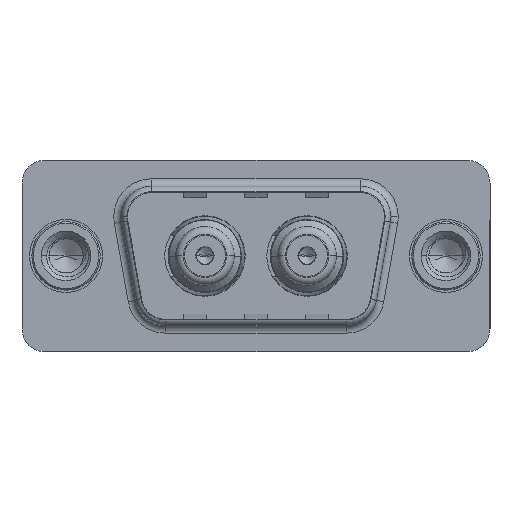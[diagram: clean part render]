
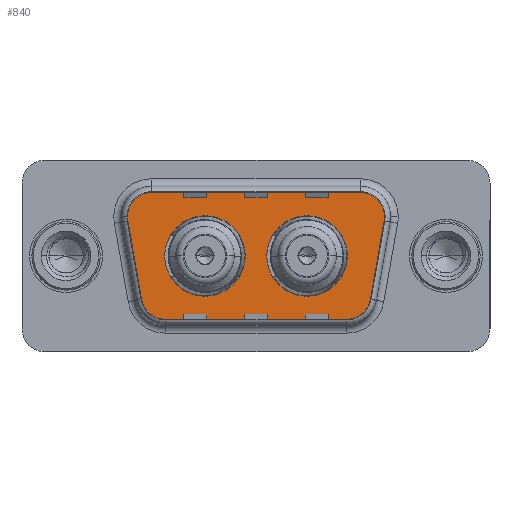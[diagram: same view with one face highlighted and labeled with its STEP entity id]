
A CAD part, top view. The second image highlights one B-rep face of the part: STEP entity #840.
In plain terms, the highlighted planar face has unit normal (0, 0, 1).
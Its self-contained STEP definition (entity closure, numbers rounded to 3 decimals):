
#60 = CARTESIAN_POINT ( 'NONE',  ( 19.564, 4.9, 0. ) ) ;
#363 = EDGE_CURVE ( 'NONE', #13739, #3804, #2081, .T. ) ;
#372 = CARTESIAN_POINT ( 'NONE',  ( 19.564, 2.9, 0. ) ) ;
#391 = ORIENTED_EDGE ( 'NONE', *, *, #12341, .F. ) ;
#644 = EDGE_CURVE ( 'NONE', #14013, #3973, #5257, .T. ) ;
#743 = VECTOR ( 'NONE', #5504, 1000. ) ;
#751 = DIRECTION ( 'NONE',  ( 0.174, -0.985, 0. ) ) ;
#840 = ADVANCED_FACE ( 'NONE', ( #3483, #7872, #12417 ), #1940, .T. ) ;
#950 = CARTESIAN_POINT ( 'NONE',  ( 6.459, -4.9, 0. ) ) ;
#1063 = CARTESIAN_POINT ( 'NONE',  ( 5.436, 4.9, 0. ) ) ;
#1158 = VECTOR ( 'NONE', #9131, 1000. ) ;
#1283 = CARTESIAN_POINT ( 'NONE',  ( 21.534, 2.553, 0. ) ) ;
#1397 = VERTEX_POINT ( 'NONE', #9898 ) ;
#1497 = DIRECTION ( 'NONE',  ( -1., 0., 0. ) ) ;
#1583 = AXIS2_PLACEMENT_3D ( 'NONE', #12875, #11607, #8328 ) ;
#1613 = AXIS2_PLACEMENT_3D ( 'NONE', #9398, #2683, #10532 ) ;
#1806 = AXIS2_PLACEMENT_3D ( 'NONE', #2772, #10595, #3891 ) ;
#1940 = PLANE ( 'NONE',  #3496 ) ;
#2081 = CIRCLE ( 'NONE', #10796, 2. ) ;
#2583 = AXIS2_PLACEMENT_3D ( 'NONE', #11770, #5081, #12899 ) ;
#2683 = DIRECTION ( 'NONE',  ( 0., 0., 1. ) ) ;
#2772 = CARTESIAN_POINT ( 'NONE',  ( 15.86, 0., 0. ) ) ;
#2928 = CARTESIAN_POINT ( 'NONE',  ( 6.49, 0., 0. ) ) ;
#2975 = CARTESIAN_POINT ( 'NONE',  ( 13.21, 0., 0. ) ) ;
#3308 = DIRECTION ( 'NONE',  ( 0., 0., 1. ) ) ;
#3353 = CIRCLE ( 'NONE', #1806, 2.65 ) ;
#3383 = LINE ( 'NONE', #12188, #743 ) ;
#3483 = FACE_BOUND ( 'NONE', #4409, .T. ) ;
#3496 = AXIS2_PLACEMENT_3D ( 'NONE', #3884, #4098, #3699 ) ;
#3699 = DIRECTION ( 'NONE',  ( 1., 0., 0. ) ) ;
#3752 = EDGE_CURVE ( 'NONE', #9953, #11164, #14135, .T. ) ;
#3804 = VERTEX_POINT ( 'NONE', #9267 ) ;
#3884 = CARTESIAN_POINT ( 'NONE',  ( 18.541, -2.9, 0. ) ) ;
#3891 = DIRECTION ( 'NONE',  ( 1., 0., 0. ) ) ;
#3973 = VERTEX_POINT ( 'NONE', #950 ) ;
#3981 = VECTOR ( 'NONE', #7996, 1000. ) ;
#4098 = DIRECTION ( 'NONE',  ( 0., 0., 1. ) ) ;
#4194 = VERTEX_POINT ( 'NONE', #10571 ) ;
#4312 = VERTEX_POINT ( 'NONE', #60 ) ;
#4409 = EDGE_LOOP ( 'NONE', ( #8155, #7057 ) ) ;
#4672 = DIRECTION ( 'NONE',  ( 0., 0., 1. ) ) ;
#4810 = EDGE_LOOP ( 'NONE', ( #6652, #8661, #8958, #5219, #11900, #6343, #7572, #9392, #8143 ) ) ;
#5014 = AXIS2_PLACEMENT_3D ( 'NONE', #13237, #6560, #14348 ) ;
#5081 = DIRECTION ( 'NONE',  ( 0., 0., 1. ) ) ;
#5219 = ORIENTED_EDGE ( 'NONE', *, *, #14343, .T. ) ;
#5249 = CARTESIAN_POINT ( 'NONE',  ( 3.466, 2.553, 0. ) ) ;
#5257 = CIRCLE ( 'NONE', #7548, 2. ) ;
#5504 = DIRECTION ( 'NONE',  ( 1., 0., 0. ) ) ;
#5770 = VERTEX_POINT ( 'NONE', #1063 ) ;
#6206 = EDGE_CURVE ( 'NONE', #1397, #14013, #9222, .T. ) ;
#6269 = VECTOR ( 'NONE', #751, 1000. ) ;
#6304 = VERTEX_POINT ( 'NONE', #7638 ) ;
#6343 = ORIENTED_EDGE ( 'NONE', *, *, #13883, .T. ) ;
#6394 = DIRECTION ( 'NONE',  ( -1., 0., 0. ) ) ;
#6417 = CARTESIAN_POINT ( 'NONE',  ( 6.459, -2.9, 0. ) ) ;
#6452 = AXIS2_PLACEMENT_3D ( 'NONE', #11360, #4672, #12480 ) ;
#6560 = DIRECTION ( 'NONE',  ( 0., 0., 1. ) ) ;
#6652 = ORIENTED_EDGE ( 'NONE', *, *, #3752, .T. ) ;
#7057 = ORIENTED_EDGE ( 'NONE', *, *, #13849, .F. ) ;
#7145 = LINE ( 'NONE', #1283, #1158 ) ;
#7276 = ORIENTED_EDGE ( 'NONE', *, *, #13219, .F. ) ;
#7540 = CARTESIAN_POINT ( 'NONE',  ( 4.489, -3.247, 0. ) ) ;
#7548 = AXIS2_PLACEMENT_3D ( 'NONE', #6417, #9700, #6394 ) ;
#7572 = ORIENTED_EDGE ( 'NONE', *, *, #6206, .T. ) ;
#7638 = CARTESIAN_POINT ( 'NONE',  ( 18.51, 0., 0. ) ) ;
#7872 = FACE_BOUND ( 'NONE', #13065, .T. ) ;
#7996 = DIRECTION ( 'NONE',  ( -1., 0., 0. ) ) ;
#8111 = CARTESIAN_POINT ( 'NONE',  ( 21.534, 2.553, 0. ) ) ;
#8143 = ORIENTED_EDGE ( 'NONE', *, *, #13095, .T. ) ;
#8155 = ORIENTED_EDGE ( 'NONE', *, *, #13400, .F. ) ;
#8236 = DIRECTION ( 'NONE',  ( 0., 0., 1. ) ) ;
#8328 = DIRECTION ( 'NONE',  ( 1., 0., 0. ) ) ;
#8661 = ORIENTED_EDGE ( 'NONE', *, *, #10889, .T. ) ;
#8838 = CIRCLE ( 'NONE', #5014, 2.65 ) ;
#8958 = ORIENTED_EDGE ( 'NONE', *, *, #363, .T. ) ;
#9131 = DIRECTION ( 'NONE',  ( 0.174, 0.985, 0. ) ) ;
#9222 = LINE ( 'NONE', #5249, #6269 ) ;
#9267 = CARTESIAN_POINT ( 'NONE',  ( 21.564, 2.9, 0. ) ) ;
#9392 = ORIENTED_EDGE ( 'NONE', *, *, #644, .T. ) ;
#9398 = CARTESIAN_POINT ( 'NONE',  ( 15.86, 0., 0. ) ) ;
#9658 = CARTESIAN_POINT ( 'NONE',  ( 20.511, -3.247, 0. ) ) ;
#9700 = DIRECTION ( 'NONE',  ( 0., 0., 1. ) ) ;
#9856 = EDGE_CURVE ( 'NONE', #4312, #5770, #10988, .T. ) ;
#9898 = CARTESIAN_POINT ( 'NONE',  ( 3.466, 2.553, 0. ) ) ;
#9953 = VERTEX_POINT ( 'NONE', #13712 ) ;
#10486 = VERTEX_POINT ( 'NONE', #2928 ) ;
#10532 = DIRECTION ( 'NONE',  ( 1., 0., 0. ) ) ;
#10561 = AXIS2_PLACEMENT_3D ( 'NONE', #372, #8236, #1497 ) ;
#10571 = CARTESIAN_POINT ( 'NONE',  ( 11.79, 0., 0. ) ) ;
#10595 = DIRECTION ( 'NONE',  ( 0., 0., 1. ) ) ;
#10796 = AXIS2_PLACEMENT_3D ( 'NONE', #11587, #3308, #11083 ) ;
#10889 = EDGE_CURVE ( 'NONE', #11164, #13739, #7145, .T. ) ;
#10909 = CIRCLE ( 'NONE', #6452, 2.65 ) ;
#10988 = LINE ( 'NONE', #11319, #3981 ) ;
#11083 = DIRECTION ( 'NONE',  ( -1., 0., 0. ) ) ;
#11164 = VERTEX_POINT ( 'NONE', #9658 ) ;
#11319 = CARTESIAN_POINT ( 'NONE',  ( 5.436, 4.9, 0. ) ) ;
#11360 = CARTESIAN_POINT ( 'NONE',  ( 9.14, 0., 0. ) ) ;
#11587 = CARTESIAN_POINT ( 'NONE',  ( 19.564, 2.9, 0. ) ) ;
#11607 = DIRECTION ( 'NONE',  ( 0., 0., 1. ) ) ;
#11770 = CARTESIAN_POINT ( 'NONE',  ( 5.436, 2.9, 0. ) ) ;
#11785 = CIRCLE ( 'NONE', #1613, 2.65 ) ;
#11900 = ORIENTED_EDGE ( 'NONE', *, *, #9856, .T. ) ;
#11935 = CIRCLE ( 'NONE', #2583, 2. ) ;
#12188 = CARTESIAN_POINT ( 'NONE',  ( 6.459, -4.9, 0. ) ) ;
#12240 = VERTEX_POINT ( 'NONE', #2975 ) ;
#12341 = EDGE_CURVE ( 'NONE', #10486, #4194, #8838, .T. ) ;
#12417 = FACE_OUTER_BOUND ( 'NONE', #4810, .T. ) ;
#12480 = DIRECTION ( 'NONE',  ( 1., 0., 0. ) ) ;
#12629 = CIRCLE ( 'NONE', #10561, 2. ) ;
#12875 = CARTESIAN_POINT ( 'NONE',  ( 18.541, -2.9, 0. ) ) ;
#12899 = DIRECTION ( 'NONE',  ( 1., 0., 0. ) ) ;
#13065 = EDGE_LOOP ( 'NONE', ( #7276, #391 ) ) ;
#13095 = EDGE_CURVE ( 'NONE', #3973, #9953, #3383, .T. ) ;
#13219 = EDGE_CURVE ( 'NONE', #4194, #10486, #10909, .T. ) ;
#13237 = CARTESIAN_POINT ( 'NONE',  ( 9.14, 0., 0. ) ) ;
#13400 = EDGE_CURVE ( 'NONE', #6304, #12240, #11785, .T. ) ;
#13712 = CARTESIAN_POINT ( 'NONE',  ( 18.541, -4.9, 0. ) ) ;
#13739 = VERTEX_POINT ( 'NONE', #8111 ) ;
#13849 = EDGE_CURVE ( 'NONE', #12240, #6304, #3353, .T. ) ;
#13883 = EDGE_CURVE ( 'NONE', #5770, #1397, #11935, .T. ) ;
#14013 = VERTEX_POINT ( 'NONE', #7540 ) ;
#14135 = CIRCLE ( 'NONE', #1583, 2. ) ;
#14343 = EDGE_CURVE ( 'NONE', #3804, #4312, #12629, .T. ) ;
#14348 = DIRECTION ( 'NONE',  ( 1., 0., 0. ) ) ;
